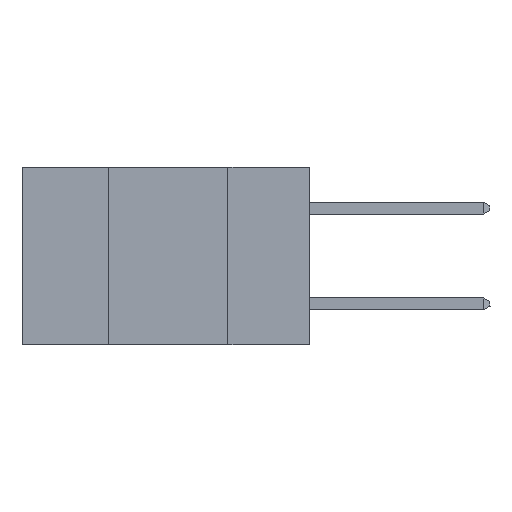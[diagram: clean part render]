
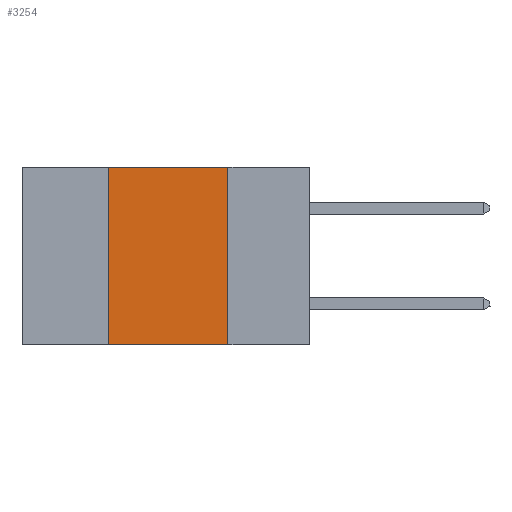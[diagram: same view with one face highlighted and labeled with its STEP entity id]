
A CAD part, left-side view. The second image highlights one B-rep face of the part: STEP entity #3254.
In plain terms, the highlighted planar face has unit normal (-1, 0, 0).
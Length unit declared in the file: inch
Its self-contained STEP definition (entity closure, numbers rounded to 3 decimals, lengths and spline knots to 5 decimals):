
#37 = VECTOR ( 'NONE', #1441, 39.37008 ) ;
#183 = EDGE_CURVE ( 'NONE', #10093, #3607, #2291, .T. ) ;
#723 = CARTESIAN_POINT ( 'NONE',  ( 0., 0.6, 0. ) ) ;
#770 = CARTESIAN_POINT ( 'NONE',  ( 0., 0.17, 0. ) ) ;
#865 = CARTESIAN_POINT ( 'NONE',  ( 0., 0.42, -0.37 ) ) ;
#1441 = DIRECTION ( 'NONE',  ( 0., -1., 0. ) ) ;
#1561 = CARTESIAN_POINT ( 'NONE',  ( 0., 0.6, 0. ) ) ;
#1681 = VECTOR ( 'NONE', #5722, 39.37008 ) ;
#1698 = VERTEX_POINT ( 'NONE', #865 ) ;
#1914 = VECTOR ( 'NONE', #10054, 39.37008 ) ;
#2291 = LINE ( 'NONE', #1561, #37 ) ;
#2447 = EDGE_CURVE ( 'NONE', #1698, #6497, #4747, .T. ) ;
#2920 = CARTESIAN_POINT ( 'NONE',  ( 0., 0.17, 0. ) ) ;
#3004 = EDGE_CURVE ( 'NONE', #3607, #6497, #6548, .T. ) ;
#3254 = ADVANCED_FACE ( 'NONE', ( #11788 ), #10924, .F. ) ;
#3607 = VERTEX_POINT ( 'NONE', #770 ) ;
#3807 = ORIENTED_EDGE ( 'NONE', *, *, #3004, .F. ) ;
#4171 = CARTESIAN_POINT ( 'NONE',  ( 0., 0.17, -0.37 ) ) ;
#4460 = DIRECTION ( 'NONE',  ( 1., 0., 0. ) ) ;
#4747 = LINE ( 'NONE', #5838, #1681 ) ;
#4930 = EDGE_CURVE ( 'NONE', #1698, #10093, #7288, .T. ) ;
#5377 = EDGE_LOOP ( 'NONE', ( #3807, #9826, #5922, #6147 ) ) ;
#5426 = AXIS2_PLACEMENT_3D ( 'NONE', #723, #4460, #8185 ) ;
#5626 = VECTOR ( 'NONE', #6666, 39.37008 ) ;
#5722 = DIRECTION ( 'NONE',  ( 0., -1., 0. ) ) ;
#5838 = CARTESIAN_POINT ( 'NONE',  ( 0., 0.6, -0.37 ) ) ;
#5922 = ORIENTED_EDGE ( 'NONE', *, *, #4930, .F. ) ;
#6147 = ORIENTED_EDGE ( 'NONE', *, *, #2447, .T. ) ;
#6497 = VERTEX_POINT ( 'NONE', #4171 ) ;
#6548 = LINE ( 'NONE', #2920, #5626 ) ;
#6666 = DIRECTION ( 'NONE',  ( 0., 0., -1. ) ) ;
#7288 = LINE ( 'NONE', #8329, #1914 ) ;
#8185 = DIRECTION ( 'NONE',  ( 0., 0., -1. ) ) ;
#8329 = CARTESIAN_POINT ( 'NONE',  ( 0., 0.42, 0. ) ) ;
#9826 = ORIENTED_EDGE ( 'NONE', *, *, #183, .F. ) ;
#10054 = DIRECTION ( 'NONE',  ( 0., 0., 1. ) ) ;
#10093 = VERTEX_POINT ( 'NONE', #11458 ) ;
#10924 = PLANE ( 'NONE',  #5426 ) ;
#11458 = CARTESIAN_POINT ( 'NONE',  ( 0., 0.42, 0. ) ) ;
#11788 = FACE_OUTER_BOUND ( 'NONE', #5377, .T. ) ;
